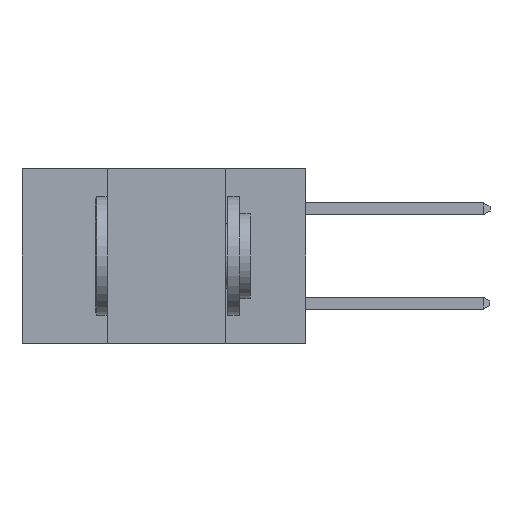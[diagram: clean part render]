
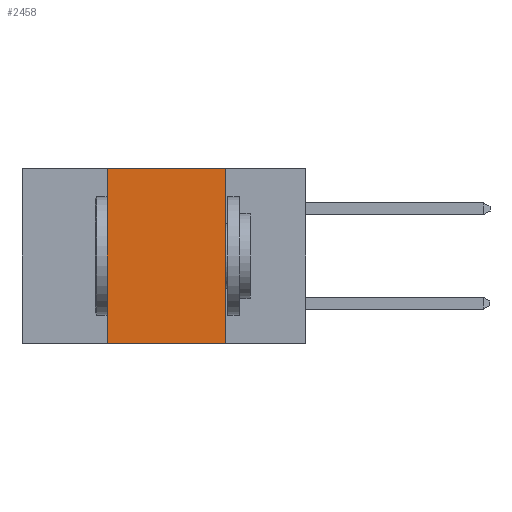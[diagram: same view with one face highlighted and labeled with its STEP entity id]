
A CAD part, left-side view. The second image highlights one B-rep face of the part: STEP entity #2458.
In plain terms, the highlighted planar face has unit normal (-1, 0, 0).
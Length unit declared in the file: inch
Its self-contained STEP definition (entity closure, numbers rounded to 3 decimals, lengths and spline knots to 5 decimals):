
#1156 = VECTOR ( 'NONE', #4023, 39.37008 ) ;
#2458 = ADVANCED_FACE ( 'NONE', ( #9524 ), #6069, .F. ) ;
#2824 = VECTOR ( 'NONE', #8527, 39.37008 ) ;
#2830 = DIRECTION ( 'NONE',  ( 0., -1., 0. ) ) ;
#3098 = LINE ( 'NONE', #4035, #1156 ) ;
#4023 = DIRECTION ( 'NONE',  ( 0., -1., 0. ) ) ;
#4035 = CARTESIAN_POINT ( 'NONE',  ( 0., 0.6, -0.37 ) ) ;
#4174 = LINE ( 'NONE', #4839, #8137 ) ;
#4199 = EDGE_CURVE ( 'NONE', #5882, #6682, #5031, .T. ) ;
#4269 = ORIENTED_EDGE ( 'NONE', *, *, #4199, .F. ) ;
#4420 = VECTOR ( 'NONE', #2830, 39.37008 ) ;
#4433 = CARTESIAN_POINT ( 'NONE',  ( 0., 0.17, 0. ) ) ;
#4472 = ORIENTED_EDGE ( 'NONE', *, *, #8720, .F. ) ;
#4726 = ORIENTED_EDGE ( 'NONE', *, *, #7173, .F. ) ;
#4839 = CARTESIAN_POINT ( 'NONE',  ( 0., 0.42, 0. ) ) ;
#4918 = DIRECTION ( 'NONE',  ( 0., 0., 1. ) ) ;
#4929 = LINE ( 'NONE', #5323, #4420 ) ;
#5031 = LINE ( 'NONE', #4433, #2824 ) ;
#5067 = ORIENTED_EDGE ( 'NONE', *, *, #7671, .T. ) ;
#5323 = CARTESIAN_POINT ( 'NONE',  ( 0., 0.6, 0. ) ) ;
#5882 = VERTEX_POINT ( 'NONE', #7837 ) ;
#6069 = PLANE ( 'NONE',  #8262 ) ;
#6682 = VERTEX_POINT ( 'NONE', #7246 ) ;
#7056 = VERTEX_POINT ( 'NONE', #9891 ) ;
#7173 = EDGE_CURVE ( 'NONE', #8772, #7056, #4174, .T. ) ;
#7246 = CARTESIAN_POINT ( 'NONE',  ( 0., 0.17, -0.37 ) ) ;
#7671 = EDGE_CURVE ( 'NONE', #8772, #6682, #3098, .T. ) ;
#7837 = CARTESIAN_POINT ( 'NONE',  ( 0., 0.17, 0. ) ) ;
#7841 = DIRECTION ( 'NONE',  ( 0., 0., -1. ) ) ;
#7853 = DIRECTION ( 'NONE',  ( 1., 0., 0. ) ) ;
#8137 = VECTOR ( 'NONE', #4918, 39.37008 ) ;
#8226 = EDGE_LOOP ( 'NONE', ( #4269, #4472, #4726, #5067 ) ) ;
#8262 = AXIS2_PLACEMENT_3D ( 'NONE', #8950, #7853, #7841 ) ;
#8489 = CARTESIAN_POINT ( 'NONE',  ( 0., 0.42, -0.37 ) ) ;
#8527 = DIRECTION ( 'NONE',  ( 0., 0., -1. ) ) ;
#8720 = EDGE_CURVE ( 'NONE', #7056, #5882, #4929, .T. ) ;
#8772 = VERTEX_POINT ( 'NONE', #8489 ) ;
#8950 = CARTESIAN_POINT ( 'NONE',  ( 0., 0.6, 0. ) ) ;
#9524 = FACE_OUTER_BOUND ( 'NONE', #8226, .T. ) ;
#9891 = CARTESIAN_POINT ( 'NONE',  ( 0., 0.42, 0. ) ) ;
